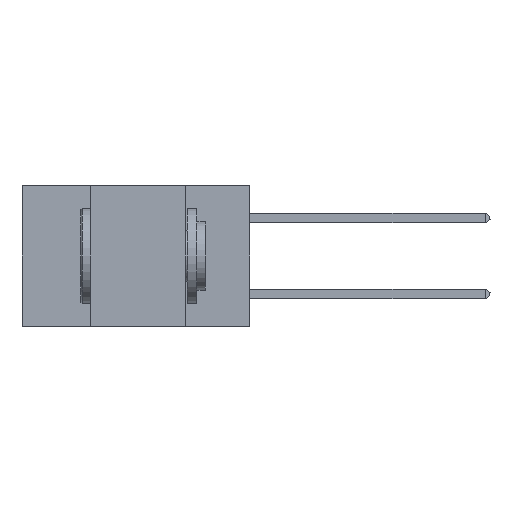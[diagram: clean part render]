
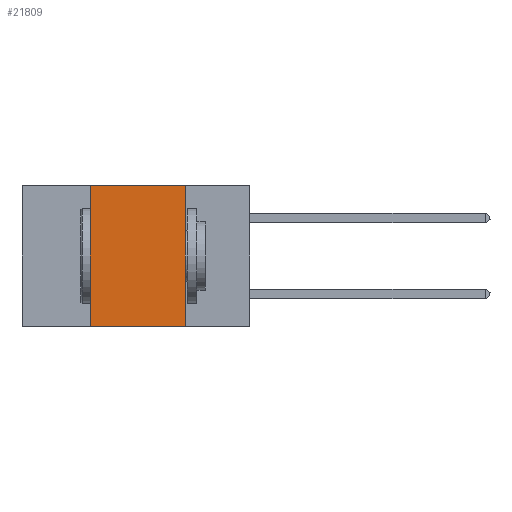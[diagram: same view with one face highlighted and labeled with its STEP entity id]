
A CAD part, left-side view. The second image highlights one B-rep face of the part: STEP entity #21809.
In plain terms, the highlighted planar face has unit normal (-1, 0, 0).
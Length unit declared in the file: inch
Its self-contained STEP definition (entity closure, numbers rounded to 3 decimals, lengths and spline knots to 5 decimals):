
#250 = ORIENTED_EDGE ( 'NONE', *, *, #6887, .F. ) ;
#487 = EDGE_CURVE ( 'NONE', #16975, #7678, #5266, .T. ) ;
#1132 = DIRECTION ( 'NONE',  ( 0., -1., 0. ) ) ;
#2214 = LINE ( 'NONE', #24716, #9823 ) ;
#4032 = VECTOR ( 'NONE', #22159, 39.37008 ) ;
#4462 = ORIENTED_EDGE ( 'NONE', *, *, #17523, .T. ) ;
#4877 = CARTESIAN_POINT ( 'NONE',  ( 0., 0.6, 0. ) ) ;
#5212 = VERTEX_POINT ( 'NONE', #12843 ) ;
#5266 = LINE ( 'NONE', #20398, #4032 ) ;
#5606 = AXIS2_PLACEMENT_3D ( 'NONE', #19435, #7775, #15442 ) ;
#5948 = CARTESIAN_POINT ( 'NONE',  ( 0., 0.42, -0.37 ) ) ;
#6535 = ORIENTED_EDGE ( 'NONE', *, *, #13580, .F. ) ;
#6887 = EDGE_CURVE ( 'NONE', #7102, #5212, #2214, .T. ) ;
#7020 = CARTESIAN_POINT ( 'NONE',  ( 0., 0.17, 0. ) ) ;
#7102 = VERTEX_POINT ( 'NONE', #5948 ) ;
#7678 = VERTEX_POINT ( 'NONE', #15001 ) ;
#7775 = DIRECTION ( 'NONE',  ( 1., 0., 0. ) ) ;
#9406 = VECTOR ( 'NONE', #1132, 39.37008 ) ;
#9823 = VECTOR ( 'NONE', #16904, 39.37008 ) ;
#11925 = VECTOR ( 'NONE', #18165, 39.37008 ) ;
#12363 = CARTESIAN_POINT ( 'NONE',  ( 0., 0.6, -0.37 ) ) ;
#12843 = CARTESIAN_POINT ( 'NONE',  ( 0., 0.42, 0. ) ) ;
#13580 = EDGE_CURVE ( 'NONE', #5212, #16975, #22569, .T. ) ;
#14999 = EDGE_LOOP ( 'NONE', ( #18189, #6535, #250, #4462 ) ) ;
#15001 = CARTESIAN_POINT ( 'NONE',  ( 0., 0.17, -0.37 ) ) ;
#15442 = DIRECTION ( 'NONE',  ( 0., 0., -1. ) ) ;
#15923 = LINE ( 'NONE', #12363, #11925 ) ;
#16904 = DIRECTION ( 'NONE',  ( 0., 0., 1. ) ) ;
#16975 = VERTEX_POINT ( 'NONE', #7020 ) ;
#17523 = EDGE_CURVE ( 'NONE', #7102, #7678, #15923, .T. ) ;
#17770 = FACE_OUTER_BOUND ( 'NONE', #14999, .T. ) ;
#18165 = DIRECTION ( 'NONE',  ( 0., -1., 0. ) ) ;
#18189 = ORIENTED_EDGE ( 'NONE', *, *, #487, .F. ) ;
#19435 = CARTESIAN_POINT ( 'NONE',  ( 0., 0.6, 0. ) ) ;
#20398 = CARTESIAN_POINT ( 'NONE',  ( 0., 0.17, 0. ) ) ;
#21809 = ADVANCED_FACE ( 'NONE', ( #17770 ), #25220, .F. ) ;
#22159 = DIRECTION ( 'NONE',  ( 0., 0., -1. ) ) ;
#22569 = LINE ( 'NONE', #4877, #9406 ) ;
#24716 = CARTESIAN_POINT ( 'NONE',  ( 0., 0.42, 0. ) ) ;
#25220 = PLANE ( 'NONE',  #5606 ) ;
